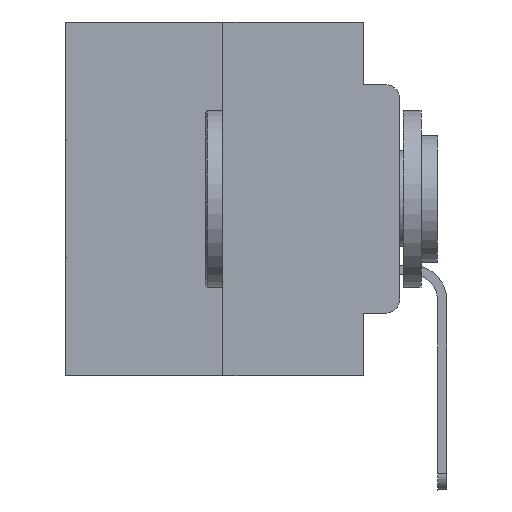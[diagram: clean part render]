
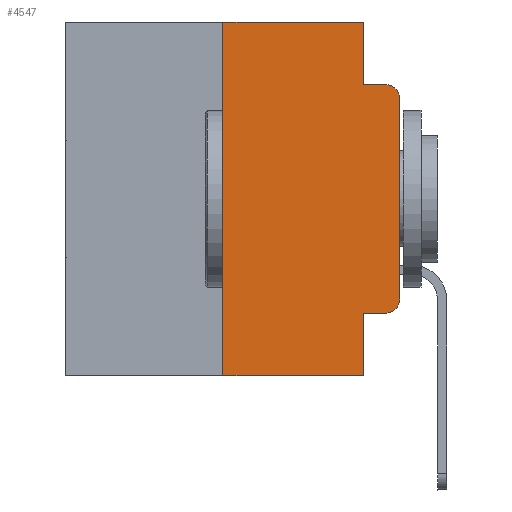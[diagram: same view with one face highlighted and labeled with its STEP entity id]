
A CAD part, left-side view. The second image highlights one B-rep face of the part: STEP entity #4547.
In plain terms, the highlighted planar face has unit normal (-1, 0, 0).
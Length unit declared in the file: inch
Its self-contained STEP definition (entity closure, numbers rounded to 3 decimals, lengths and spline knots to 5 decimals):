
#72 = LINE ( 'NONE', #8600, #5343 ) ;
#182 = VECTOR ( 'NONE', #8092, 39.37008 ) ;
#342 = EDGE_CURVE ( 'NONE', #13635, #19945, #1576, .T. ) ;
#1099 = EDGE_CURVE ( 'NONE', #13706, #4308, #13816, .T. ) ;
#1242 = DIRECTION ( 'NONE',  ( 0., 0., 1. ) ) ;
#1576 = LINE ( 'NONE', #10098, #27285 ) ;
#1681 = LINE ( 'NONE', #6278, #182 ) ;
#2000 = CIRCLE ( 'NONE', #17630, 0.02 ) ;
#2618 = LINE ( 'NONE', #19539, #19312 ) ;
#3476 = CARTESIAN_POINT ( 'NONE',  ( 0., 0.051, -0.0885 ) ) ;
#3607 = ORIENTED_EDGE ( 'NONE', *, *, #342, .T. ) ;
#3952 = VERTEX_POINT ( 'NONE', #18931 ) ;
#4308 = VERTEX_POINT ( 'NONE', #11226 ) ;
#4547 = ADVANCED_FACE ( 'NONE', ( #12610 ), #21684, .F. ) ;
#4865 = CARTESIAN_POINT ( 'NONE',  ( 0., 0.051, 0. ) ) ;
#4868 = EDGE_CURVE ( 'NONE', #25336, #11671, #25179, .T. ) ;
#4941 = VECTOR ( 'NONE', #1242, 39.37008 ) ;
#5124 = ORIENTED_EDGE ( 'NONE', *, *, #11813, .F. ) ;
#5343 = VECTOR ( 'NONE', #6496, 39.37008 ) ;
#5348 = CARTESIAN_POINT ( 'NONE',  ( 0., 0.02, -0.1085 ) ) ;
#6278 = CARTESIAN_POINT ( 'NONE',  ( 0., 0.051, -0.4115 ) ) ;
#6496 = DIRECTION ( 'NONE',  ( 0., -1., 0. ) ) ;
#7505 = CARTESIAN_POINT ( 'NONE',  ( 0., 0.051, 0. ) ) ;
#8092 = DIRECTION ( 'NONE',  ( 0., -1., 0. ) ) ;
#8396 = CARTESIAN_POINT ( 'NONE',  ( 0., 0.473, 0. ) ) ;
#8600 = CARTESIAN_POINT ( 'NONE',  ( 0., 0.473, -0.5 ) ) ;
#8647 = VECTOR ( 'NONE', #9775, 39.37008 ) ;
#9330 = CARTESIAN_POINT ( 'NONE',  ( 0., 0.25, 0. ) ) ;
#9775 = DIRECTION ( 'NONE',  ( 0., -1., 0. ) ) ;
#9972 = CARTESIAN_POINT ( 'NONE',  ( 0., 0.02, -0.4115 ) ) ;
#10098 = CARTESIAN_POINT ( 'NONE',  ( 0., 0., 0. ) ) ;
#10103 = CARTESIAN_POINT ( 'NONE',  ( 0., 0., -0.1085 ) ) ;
#10147 = CARTESIAN_POINT ( 'NONE',  ( 0., 0.02, -0.3915 ) ) ;
#10277 = DIRECTION ( 'NONE',  ( 0., 0., -1. ) ) ;
#10769 = DIRECTION ( 'NONE',  ( 0., 0., -1. ) ) ;
#10772 = EDGE_CURVE ( 'NONE', #19518, #11469, #27500, .T. ) ;
#10810 = AXIS2_PLACEMENT_3D ( 'NONE', #8396, #17216, #10769 ) ;
#11021 = EDGE_CURVE ( 'NONE', #3952, #4308, #72, .T. ) ;
#11226 = CARTESIAN_POINT ( 'NONE',  ( 0., 0.051, -0.5 ) ) ;
#11469 = VERTEX_POINT ( 'NONE', #19479 ) ;
#11504 = ORIENTED_EDGE ( 'NONE', *, *, #13678, .T. ) ;
#11671 = VERTEX_POINT ( 'NONE', #4865 ) ;
#11786 = ORIENTED_EDGE ( 'NONE', *, *, #10772, .F. ) ;
#11813 = EDGE_CURVE ( 'NONE', #3952, #25336, #24584, .T. ) ;
#11837 = ORIENTED_EDGE ( 'NONE', *, *, #1099, .F. ) ;
#11931 = DIRECTION ( 'NONE',  ( 0., 0., -1. ) ) ;
#12105 = CARTESIAN_POINT ( 'NONE',  ( 0., 0., -0.3915 ) ) ;
#12115 = DIRECTION ( 'NONE',  ( 0., -1., 0. ) ) ;
#12395 = DIRECTION ( 'NONE',  ( -1., 0., 0. ) ) ;
#12610 = FACE_OUTER_BOUND ( 'NONE', #20009, .T. ) ;
#12880 = VERTEX_POINT ( 'NONE', #9972 ) ;
#12963 = DIRECTION ( 'NONE',  ( 0., 0., -1. ) ) ;
#13116 = ORIENTED_EDGE ( 'NONE', *, *, #19780, .T. ) ;
#13394 = VECTOR ( 'NONE', #12115, 39.37008 ) ;
#13635 = VERTEX_POINT ( 'NONE', #12105 ) ;
#13678 = EDGE_CURVE ( 'NONE', #12880, #13635, #26862, .T. ) ;
#13706 = VERTEX_POINT ( 'NONE', #23145 ) ;
#13816 = LINE ( 'NONE', #7505, #21461 ) ;
#15568 = DIRECTION ( 'NONE',  ( -1., 0., 0. ) ) ;
#15698 = ORIENTED_EDGE ( 'NONE', *, *, #11021, .T. ) ;
#17216 = DIRECTION ( 'NONE',  ( 1., 0., 0. ) ) ;
#17630 = AXIS2_PLACEMENT_3D ( 'NONE', #5348, #15568, #11931 ) ;
#17972 = EDGE_CURVE ( 'NONE', #13706, #12880, #1681, .T. ) ;
#18321 = ORIENTED_EDGE ( 'NONE', *, *, #17972, .T. ) ;
#18931 = CARTESIAN_POINT ( 'NONE',  ( 0., 0.25, -0.5 ) ) ;
#19312 = VECTOR ( 'NONE', #12963, 39.37008 ) ;
#19479 = CARTESIAN_POINT ( 'NONE',  ( 0., 0.02, -0.0885 ) ) ;
#19518 = VERTEX_POINT ( 'NONE', #3476 ) ;
#19539 = CARTESIAN_POINT ( 'NONE',  ( 0., 0.051, 0. ) ) ;
#19780 = EDGE_CURVE ( 'NONE', #19945, #11469, #2000, .T. ) ;
#19945 = VERTEX_POINT ( 'NONE', #10103 ) ;
#20009 = EDGE_LOOP ( 'NONE', ( #3607, #13116, #11786, #24651, #21384, #5124, #15698, #11837, #18321, #11504 ) ) ;
#21384 = ORIENTED_EDGE ( 'NONE', *, *, #4868, .F. ) ;
#21461 = VECTOR ( 'NONE', #22337, 39.37008 ) ;
#21684 = PLANE ( 'NONE',  #10810 ) ;
#22337 = DIRECTION ( 'NONE',  ( 0., 0., -1. ) ) ;
#23145 = CARTESIAN_POINT ( 'NONE',  ( 0., 0.051, -0.4115 ) ) ;
#24187 = AXIS2_PLACEMENT_3D ( 'NONE', #10147, #12395, #10277 ) ;
#24584 = LINE ( 'NONE', #9330, #4941 ) ;
#24651 = ORIENTED_EDGE ( 'NONE', *, *, #26994, .F. ) ;
#24886 = CARTESIAN_POINT ( 'NONE',  ( 0., 0.473, 0. ) ) ;
#25179 = LINE ( 'NONE', #24886, #8647 ) ;
#25336 = VERTEX_POINT ( 'NONE', #26254 ) ;
#26254 = CARTESIAN_POINT ( 'NONE',  ( 0., 0.25, 0. ) ) ;
#26862 = CIRCLE ( 'NONE', #24187, 0.02 ) ;
#26994 = EDGE_CURVE ( 'NONE', #11671, #19518, #2618, .T. ) ;
#27221 = CARTESIAN_POINT ( 'NONE',  ( 0., 0.051, -0.0885 ) ) ;
#27285 = VECTOR ( 'NONE', #27293, 39.37008 ) ;
#27293 = DIRECTION ( 'NONE',  ( 0., 0., 1. ) ) ;
#27500 = LINE ( 'NONE', #27221, #13394 ) ;
